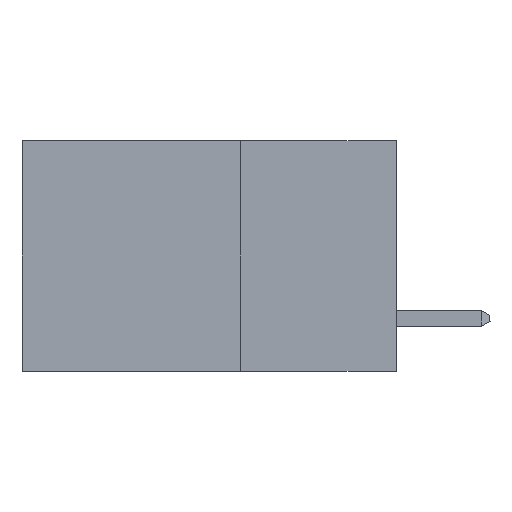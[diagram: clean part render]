
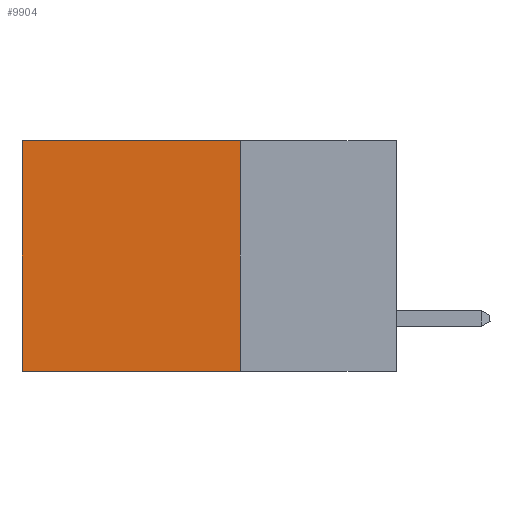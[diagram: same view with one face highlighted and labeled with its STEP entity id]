
A CAD part, left-side view. The second image highlights one B-rep face of the part: STEP entity #9904.
In plain terms, the highlighted planar face has unit normal (-1, 0, 0).
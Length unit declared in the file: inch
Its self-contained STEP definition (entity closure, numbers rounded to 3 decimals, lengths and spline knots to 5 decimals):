
#191 = VECTOR ( 'NONE', #5403, 39.37008 ) ;
#636 = VECTOR ( 'NONE', #6603, 39.37008 ) ;
#915 = FACE_OUTER_BOUND ( 'NONE', #5698, .T. ) ;
#1583 = DIRECTION ( 'NONE',  ( 1., 0., 0. ) ) ;
#2438 = LINE ( 'NONE', #9150, #7388 ) ;
#2521 = CARTESIAN_POINT ( 'NONE',  ( 0.298, 0.25, 0. ) ) ;
#2797 = CARTESIAN_POINT ( 'NONE',  ( 0.298, 0.25, 0. ) ) ;
#2811 = LINE ( 'NONE', #7658, #191 ) ;
#2912 = ORIENTED_EDGE ( 'NONE', *, *, #12416, .F. ) ;
#3175 = DIRECTION ( 'NONE',  ( 0., 0., -1. ) ) ;
#3402 = LINE ( 'NONE', #5748, #10644 ) ;
#3559 = DIRECTION ( 'NONE',  ( 0., 0., -1. ) ) ;
#3655 = EDGE_CURVE ( 'NONE', #7222, #8069, #2438, .T. ) ;
#3711 = CARTESIAN_POINT ( 'NONE',  ( 0.298, 0.6, -0.37 ) ) ;
#4586 = ORIENTED_EDGE ( 'NONE', *, *, #9174, .F. ) ;
#4913 = AXIS2_PLACEMENT_3D ( 'NONE', #2521, #1583, #3559 ) ;
#5403 = DIRECTION ( 'NONE',  ( 0., 1., 0. ) ) ;
#5698 = EDGE_LOOP ( 'NONE', ( #6227, #4586, #2912, #7139 ) ) ;
#5748 = CARTESIAN_POINT ( 'NONE',  ( 0.298, 0.25, -0.37 ) ) ;
#6227 = ORIENTED_EDGE ( 'NONE', *, *, #3655, .T. ) ;
#6496 = LINE ( 'NONE', #2797, #636 ) ;
#6603 = DIRECTION ( 'NONE',  ( 0., 0., -1. ) ) ;
#7139 = ORIENTED_EDGE ( 'NONE', *, *, #11410, .T. ) ;
#7222 = VERTEX_POINT ( 'NONE', #11081 ) ;
#7388 = VECTOR ( 'NONE', #3175, 39.37008 ) ;
#7658 = CARTESIAN_POINT ( 'NONE',  ( 0.298, 0.25, 0. ) ) ;
#8069 = VERTEX_POINT ( 'NONE', #3711 ) ;
#9150 = CARTESIAN_POINT ( 'NONE',  ( 0.298, 0.6, 0. ) ) ;
#9174 = EDGE_CURVE ( 'NONE', #12639, #8069, #3402, .T. ) ;
#9904 = ADVANCED_FACE ( 'NONE', ( #915 ), #12314, .F. ) ;
#10644 = VECTOR ( 'NONE', #12655, 39.37008 ) ;
#10687 = CARTESIAN_POINT ( 'NONE',  ( 0.298, 0.25, 0. ) ) ;
#11081 = CARTESIAN_POINT ( 'NONE',  ( 0.298, 0.6, 0. ) ) ;
#11410 = EDGE_CURVE ( 'NONE', #12457, #7222, #2811, .T. ) ;
#12142 = CARTESIAN_POINT ( 'NONE',  ( 0.298, 0.25, -0.37 ) ) ;
#12314 = PLANE ( 'NONE',  #4913 ) ;
#12416 = EDGE_CURVE ( 'NONE', #12457, #12639, #6496, .T. ) ;
#12457 = VERTEX_POINT ( 'NONE', #10687 ) ;
#12639 = VERTEX_POINT ( 'NONE', #12142 ) ;
#12655 = DIRECTION ( 'NONE',  ( 0., 1., 0. ) ) ;
